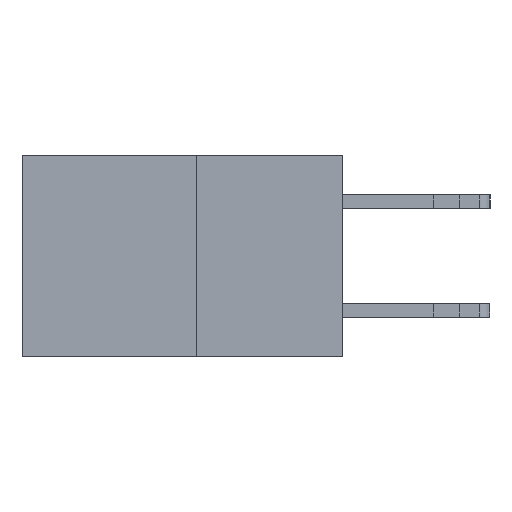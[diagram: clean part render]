
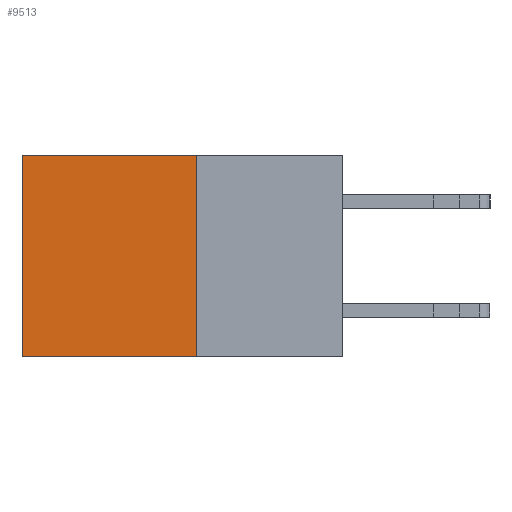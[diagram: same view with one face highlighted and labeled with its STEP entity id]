
A CAD part, left-side view. The second image highlights one B-rep face of the part: STEP entity #9513.
In plain terms, the highlighted planar face has unit normal (-1, 0, 0).
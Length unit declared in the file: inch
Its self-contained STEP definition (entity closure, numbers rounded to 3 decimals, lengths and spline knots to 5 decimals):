
#1937 = EDGE_LOOP ( 'NONE', ( #4068, #8777, #11229, #2528 ) ) ;
#1976 = AXIS2_PLACEMENT_3D ( 'NONE', #2800, #12473, #4229 ) ;
#2269 = EDGE_CURVE ( 'NONE', #4211, #17080, #7817, .T. ) ;
#2528 = ORIENTED_EDGE ( 'NONE', *, *, #6251, .T. ) ;
#2644 = EDGE_CURVE ( 'NONE', #4605, #4686, #3286, .T. ) ;
#2800 = CARTESIAN_POINT ( 'NONE',  ( 0.277, 0.27, -0.37 ) ) ;
#2937 = VECTOR ( 'NONE', #4314, 39.37008 ) ;
#3195 = VECTOR ( 'NONE', #13558, 39.37008 ) ;
#3286 = LINE ( 'NONE', #10393, #10245 ) ;
#4068 = ORIENTED_EDGE ( 'NONE', *, *, #2269, .T. ) ;
#4211 = VERTEX_POINT ( 'NONE', #9839 ) ;
#4229 = DIRECTION ( 'NONE',  ( 0., 0., -1. ) ) ;
#4314 = DIRECTION ( 'NONE',  ( 0., 1., 0. ) ) ;
#4336 = VECTOR ( 'NONE', #5707, 39.37008 ) ;
#4605 = VERTEX_POINT ( 'NONE', #6419 ) ;
#4686 = VERTEX_POINT ( 'NONE', #17347 ) ;
#5707 = DIRECTION ( 'NONE',  ( 0., 1., 0. ) ) ;
#6251 = EDGE_CURVE ( 'NONE', #4605, #4211, #10336, .T. ) ;
#6419 = CARTESIAN_POINT ( 'NONE',  ( 0.277, 0.27, 0. ) ) ;
#7817 = LINE ( 'NONE', #10978, #3195 ) ;
#8777 = ORIENTED_EDGE ( 'NONE', *, *, #15719, .F. ) ;
#9513 = ADVANCED_FACE ( 'NONE', ( #13004 ), #11103, .F. ) ;
#9839 = CARTESIAN_POINT ( 'NONE',  ( 0.277, 0.59, 0. ) ) ;
#10245 = VECTOR ( 'NONE', #12822, 39.37008 ) ;
#10336 = LINE ( 'NONE', #16543, #2937 ) ;
#10393 = CARTESIAN_POINT ( 'NONE',  ( 0.277, 0.27, -0.37 ) ) ;
#10978 = CARTESIAN_POINT ( 'NONE',  ( 0.277, 0.59, -0.37 ) ) ;
#11103 = PLANE ( 'NONE',  #1976 ) ;
#11229 = ORIENTED_EDGE ( 'NONE', *, *, #2644, .F. ) ;
#12473 = DIRECTION ( 'NONE',  ( 1., 0., 0. ) ) ;
#12822 = DIRECTION ( 'NONE',  ( 0., 0., -1. ) ) ;
#13004 = FACE_OUTER_BOUND ( 'NONE', #1937, .T. ) ;
#13558 = DIRECTION ( 'NONE',  ( 0., 0., -1. ) ) ;
#13867 = CARTESIAN_POINT ( 'NONE',  ( 0.277, 0.27, -0.37 ) ) ;
#14373 = LINE ( 'NONE', #13867, #4336 ) ;
#15719 = EDGE_CURVE ( 'NONE', #4686, #17080, #14373, .T. ) ;
#16543 = CARTESIAN_POINT ( 'NONE',  ( 0.277, 0.27, 0. ) ) ;
#17080 = VERTEX_POINT ( 'NONE', #17173 ) ;
#17173 = CARTESIAN_POINT ( 'NONE',  ( 0.277, 0.59, -0.37 ) ) ;
#17347 = CARTESIAN_POINT ( 'NONE',  ( 0.277, 0.27, -0.37 ) ) ;
